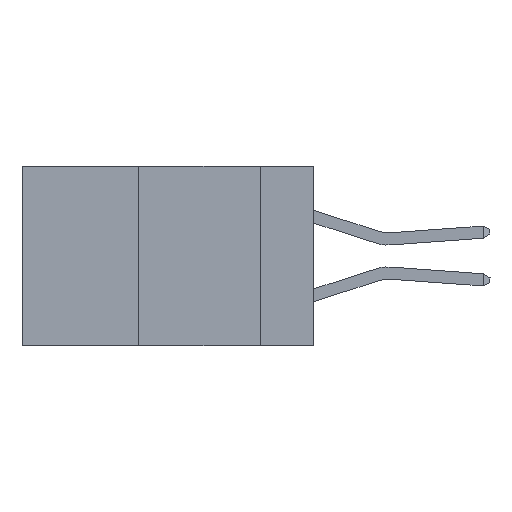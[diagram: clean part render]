
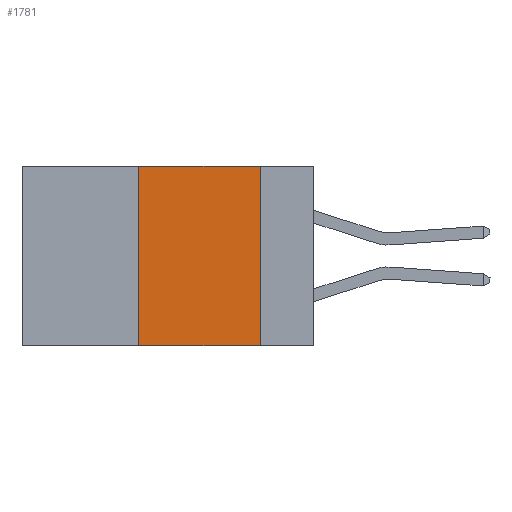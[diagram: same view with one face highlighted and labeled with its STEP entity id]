
A CAD part, left-side view. The second image highlights one B-rep face of the part: STEP entity #1781.
In plain terms, the highlighted planar face has unit normal (-1, 0, 0).
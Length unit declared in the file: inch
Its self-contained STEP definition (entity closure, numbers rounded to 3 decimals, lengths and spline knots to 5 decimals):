
#449 = FACE_OUTER_BOUND ( 'NONE', #13155, .T. ) ;
#654 = CARTESIAN_POINT ( 'NONE',  ( 0., 0.36, -0.37 ) ) ;
#1781 = ADVANCED_FACE ( 'NONE', ( #449 ), #16125, .F. ) ;
#1936 = VERTEX_POINT ( 'NONE', #6297 ) ;
#2629 = ORIENTED_EDGE ( 'NONE', *, *, #21657, .F. ) ;
#3390 = EDGE_CURVE ( 'NONE', #11471, #1936, #21953, .T. ) ;
#3435 = LINE ( 'NONE', #21046, #7486 ) ;
#3578 = EDGE_CURVE ( 'NONE', #11471, #21225, #3435, .T. ) ;
#4165 = CARTESIAN_POINT ( 'NONE',  ( 0., 0.11, 0. ) ) ;
#5076 = DIRECTION ( 'NONE',  ( 0., -1., 0. ) ) ;
#5273 = VECTOR ( 'NONE', #9263, 39.37008 ) ;
#5716 = CARTESIAN_POINT ( 'NONE',  ( 0., 0.11, 0. ) ) ;
#5804 = DIRECTION ( 'NONE',  ( 0., 0., -1. ) ) ;
#5832 = LINE ( 'NONE', #5716, #9295 ) ;
#6113 = ORIENTED_EDGE ( 'NONE', *, *, #17300, .F. ) ;
#6297 = CARTESIAN_POINT ( 'NONE',  ( 0., 0.36, 0. ) ) ;
#7222 = CARTESIAN_POINT ( 'NONE',  ( 0., 0.6, 0. ) ) ;
#7486 = VECTOR ( 'NONE', #5076, 39.37008 ) ;
#9263 = DIRECTION ( 'NONE',  ( 0., -1., 0. ) ) ;
#9295 = VECTOR ( 'NONE', #5804, 39.37008 ) ;
#10637 = VECTOR ( 'NONE', #24537, 39.37008 ) ;
#10857 = CARTESIAN_POINT ( 'NONE',  ( 0., 0.36, 0. ) ) ;
#11471 = VERTEX_POINT ( 'NONE', #654 ) ;
#13155 = EDGE_LOOP ( 'NONE', ( #2629, #6113, #24899, #24259 ) ) ;
#16125 = PLANE ( 'NONE',  #17736 ) ;
#17111 = VERTEX_POINT ( 'NONE', #4165 ) ;
#17300 = EDGE_CURVE ( 'NONE', #1936, #17111, #20965, .T. ) ;
#17736 = AXIS2_PLACEMENT_3D ( 'NONE', #22172, #22093, #18046 ) ;
#18046 = DIRECTION ( 'NONE',  ( 0., 0., -1. ) ) ;
#20965 = LINE ( 'NONE', #7222, #5273 ) ;
#21046 = CARTESIAN_POINT ( 'NONE',  ( 0., 0.6, -0.37 ) ) ;
#21225 = VERTEX_POINT ( 'NONE', #22485 ) ;
#21657 = EDGE_CURVE ( 'NONE', #17111, #21225, #5832, .T. ) ;
#21953 = LINE ( 'NONE', #10857, #10637 ) ;
#22093 = DIRECTION ( 'NONE',  ( 1., 0., 0. ) ) ;
#22172 = CARTESIAN_POINT ( 'NONE',  ( 0., 0.6, 0. ) ) ;
#22485 = CARTESIAN_POINT ( 'NONE',  ( 0., 0.11, -0.37 ) ) ;
#24259 = ORIENTED_EDGE ( 'NONE', *, *, #3578, .T. ) ;
#24537 = DIRECTION ( 'NONE',  ( 0., 0., 1. ) ) ;
#24899 = ORIENTED_EDGE ( 'NONE', *, *, #3390, .F. ) ;
